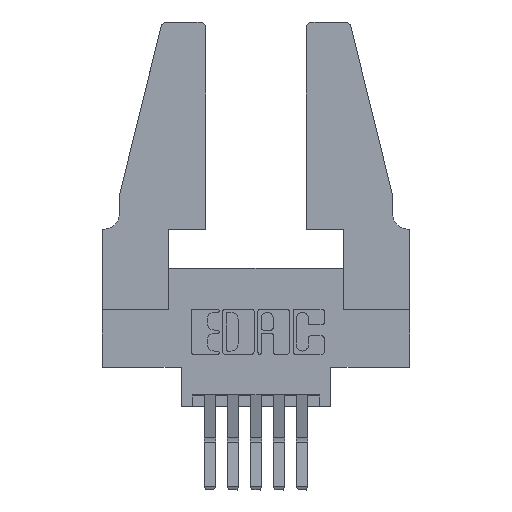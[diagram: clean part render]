
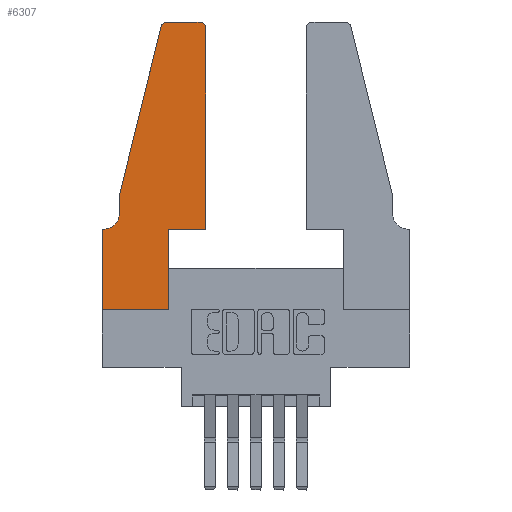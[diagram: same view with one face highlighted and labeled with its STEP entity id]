
A CAD part, top view. The second image highlights one B-rep face of the part: STEP entity #6307.
In plain terms, the highlighted planar face has unit normal (0, 0, 1).
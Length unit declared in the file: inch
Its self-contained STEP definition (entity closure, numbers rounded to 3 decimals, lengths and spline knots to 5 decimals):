
#401 = LINE ( 'NONE', #994, #9424 ) ;
#430 = VERTEX_POINT ( 'NONE', #8927 ) ;
#494 = VERTEX_POINT ( 'NONE', #2024 ) ;
#522 = CARTESIAN_POINT ( 'NONE',  ( 0.0755, 0.5, 0.37 ) ) ;
#534 = EDGE_CURVE ( 'NONE', #494, #732, #2366, .T. ) ;
#602 = CARTESIAN_POINT ( 'NONE',  ( 0.0755, 0.5, 0.37 ) ) ;
#732 = VERTEX_POINT ( 'NONE', #6600 ) ;
#889 = CARTESIAN_POINT ( 'NONE',  ( 0., 0., 0.37 ) ) ;
#952 = EDGE_CURVE ( 'NONE', #11225, #2817, #4703, .T. ) ;
#994 = CARTESIAN_POINT ( 'NONE',  ( 0.2605, 1.25, 0.37 ) ) ;
#1183 = CARTESIAN_POINT ( 'NONE',  ( 0., 0.35, 0.37 ) ) ;
#1318 = EDGE_CURVE ( 'NONE', #732, #4500, #10304, .T. ) ;
#1657 = ORIENTED_EDGE ( 'NONE', *, *, #7045, .T. ) ;
#1787 = DIRECTION ( 'NONE',  ( -1., 0., 0. ) ) ;
#1921 = DIRECTION ( 'NONE',  ( -1., 0., 0. ) ) ;
#1970 = VECTOR ( 'NONE', #2753, 39.37008 ) ;
#2024 = CARTESIAN_POINT ( 'NONE',  ( 0.0055, 0.35, 0.37 ) ) ;
#2245 = ORIENTED_EDGE ( 'NONE', *, *, #534, .T. ) ;
#2366 = LINE ( 'NONE', #7847, #11235 ) ;
#2430 = DIRECTION ( 'NONE',  ( 1., 0., 0. ) ) ;
#2753 = DIRECTION ( 'NONE',  ( 1., 0., 0. ) ) ;
#2759 = VERTEX_POINT ( 'NONE', #7954 ) ;
#2770 = CARTESIAN_POINT ( 'NONE',  ( 0.4505, 1.22, 0.37 ) ) ;
#2807 = AXIS2_PLACEMENT_3D ( 'NONE', #8177, #3059, #9028 ) ;
#2809 = ORIENTED_EDGE ( 'NONE', *, *, #9688, .T. ) ;
#2817 = VERTEX_POINT ( 'NONE', #7139 ) ;
#2929 = LINE ( 'NONE', #602, #4438 ) ;
#2940 = LINE ( 'NONE', #3236, #4973 ) ;
#3044 = DIRECTION ( 'NONE',  ( 0., 0., 1. ) ) ;
#3059 = DIRECTION ( 'NONE',  ( 0., 0., -1. ) ) ;
#3088 = DIRECTION ( 'NONE',  ( 0., 0., 1. ) ) ;
#3107 = LINE ( 'NONE', #4542, #5120 ) ;
#3236 = CARTESIAN_POINT ( 'NONE',  ( 0.2865, 0.35, 0.37 ) ) ;
#3252 = DIRECTION ( 'NONE',  ( 0., 1., 0. ) ) ;
#3321 = DIRECTION ( 'NONE',  ( -0.239, -0.971, 0. ) ) ;
#3409 = EDGE_CURVE ( 'NONE', #2759, #3925, #9166, .T. ) ;
#3623 = FACE_OUTER_BOUND ( 'NONE', #10548, .T. ) ;
#3715 = CARTESIAN_POINT ( 'NONE',  ( 0., 0., 0.37 ) ) ;
#3820 = ORIENTED_EDGE ( 'NONE', *, *, #952, .T. ) ;
#3827 = EDGE_CURVE ( 'NONE', #7275, #11225, #401, .T. ) ;
#3925 = VERTEX_POINT ( 'NONE', #2770 ) ;
#4138 = EDGE_CURVE ( 'NONE', #430, #9712, #2940, .T. ) ;
#4382 = CARTESIAN_POINT ( 'NONE',  ( 0.0755, 0.5, 0.37 ) ) ;
#4438 = VECTOR ( 'NONE', #7618, 39.37008 ) ;
#4500 = VERTEX_POINT ( 'NONE', #9816 ) ;
#4542 = CARTESIAN_POINT ( 'NONE',  ( 0.4505, 0.35, 0.37 ) ) ;
#4644 = VECTOR ( 'NONE', #9183, 39.37008 ) ;
#4703 = CIRCLE ( 'NONE', #6065, 0.03 ) ;
#4973 = VECTOR ( 'NONE', #3252, 39.37008 ) ;
#5120 = VECTOR ( 'NONE', #9648, 39.37008 ) ;
#5141 = CARTESIAN_POINT ( 'NONE',  ( 0.284, 1.22, 0.37 ) ) ;
#5285 = EDGE_CURVE ( 'NONE', #6671, #7124, #2929, .T. ) ;
#5353 = CARTESIAN_POINT ( 'NONE',  ( 0.4505, 0.35, 0.37 ) ) ;
#5599 = CIRCLE ( 'NONE', #10976, 0.03 ) ;
#5601 = PLANE ( 'NONE',  #10428 ) ;
#5956 = CARTESIAN_POINT ( 'NONE',  ( 0.0755, 0.42, 0.37 ) ) ;
#6065 = AXIS2_PLACEMENT_3D ( 'NONE', #5141, #9351, #2430 ) ;
#6307 = ADVANCED_FACE ( 'NONE', ( #3623 ), #5601, .T. ) ;
#6325 = EDGE_CURVE ( 'NONE', #3925, #7275, #5599, .T. ) ;
#6600 = CARTESIAN_POINT ( 'NONE',  ( 0., 0.35, 0.37 ) ) ;
#6671 = VERTEX_POINT ( 'NONE', #4382 ) ;
#6820 = ORIENTED_EDGE ( 'NONE', *, *, #1318, .T. ) ;
#6933 = CARTESIAN_POINT ( 'NONE',  ( 0.4205, 1.25, 0.37 ) ) ;
#7045 = EDGE_CURVE ( 'NONE', #2817, #6671, #11178, .T. ) ;
#7097 = ORIENTED_EDGE ( 'NONE', *, *, #4138, .T. ) ;
#7124 = VERTEX_POINT ( 'NONE', #5956 ) ;
#7139 = CARTESIAN_POINT ( 'NONE',  ( 0.25487, 1.22718, 0.37 ) ) ;
#7272 = CARTESIAN_POINT ( 'NONE',  ( 0.284, 1.25, 0.37 ) ) ;
#7275 = VERTEX_POINT ( 'NONE', #6933 ) ;
#7373 = ORIENTED_EDGE ( 'NONE', *, *, #3409, .T. ) ;
#7618 = DIRECTION ( 'NONE',  ( 0., -1., 0. ) ) ;
#7630 = ORIENTED_EDGE ( 'NONE', *, *, #6325, .T. ) ;
#7812 = CIRCLE ( 'NONE', #2807, 0.07 ) ;
#7847 = CARTESIAN_POINT ( 'NONE',  ( 0.0755, 0.35, 0.37 ) ) ;
#7954 = CARTESIAN_POINT ( 'NONE',  ( 0.4505, 0.35, 0.37 ) ) ;
#8007 = VECTOR ( 'NONE', #9663, 39.37008 ) ;
#8035 = ORIENTED_EDGE ( 'NONE', *, *, #3827, .T. ) ;
#8038 = EDGE_CURVE ( 'NONE', #7124, #494, #7812, .T. ) ;
#8177 = CARTESIAN_POINT ( 'NONE',  ( 0.0055, 0.42, 0.37 ) ) ;
#8203 = CARTESIAN_POINT ( 'NONE',  ( 0.4205, 1.22, 0.37 ) ) ;
#8839 = ORIENTED_EDGE ( 'NONE', *, *, #8038, .T. ) ;
#8903 = VECTOR ( 'NONE', #3321, 39.37008 ) ;
#8927 = CARTESIAN_POINT ( 'NONE',  ( 0.2865, 0., 0.37 ) ) ;
#9020 = DIRECTION ( 'NONE',  ( 1., 0., 0. ) ) ;
#9028 = DIRECTION ( 'NONE',  ( -1., 0., 0. ) ) ;
#9056 = DIRECTION ( 'NONE',  ( 1., 0., 0. ) ) ;
#9109 = ORIENTED_EDGE ( 'NONE', *, *, #10422, .T. ) ;
#9166 = LINE ( 'NONE', #5353, #4644 ) ;
#9183 = DIRECTION ( 'NONE',  ( 0., 1., 0. ) ) ;
#9351 = DIRECTION ( 'NONE',  ( 0., 0., 1. ) ) ;
#9424 = VECTOR ( 'NONE', #1921, 39.37008 ) ;
#9648 = DIRECTION ( 'NONE',  ( 1., 0., 0. ) ) ;
#9663 = DIRECTION ( 'NONE',  ( 0., -1., 0. ) ) ;
#9687 = CARTESIAN_POINT ( 'NONE',  ( 0.2865, 0.35, 0.37 ) ) ;
#9688 = EDGE_CURVE ( 'NONE', #9712, #2759, #3107, .T. ) ;
#9712 = VERTEX_POINT ( 'NONE', #9687 ) ;
#9816 = CARTESIAN_POINT ( 'NONE',  ( 0., 0., 0.37 ) ) ;
#10304 = LINE ( 'NONE', #3715, #8007 ) ;
#10422 = EDGE_CURVE ( 'NONE', #4500, #430, #11131, .T. ) ;
#10428 = AXIS2_PLACEMENT_3D ( 'NONE', #1183, #3044, #9020 ) ;
#10548 = EDGE_LOOP ( 'NONE', ( #8035, #3820, #1657, #10859, #8839, #2245, #6820, #9109, #7097, #2809, #7373, #7630 ) ) ;
#10859 = ORIENTED_EDGE ( 'NONE', *, *, #5285, .T. ) ;
#10976 = AXIS2_PLACEMENT_3D ( 'NONE', #8203, #3088, #9056 ) ;
#11131 = LINE ( 'NONE', #889, #1970 ) ;
#11178 = LINE ( 'NONE', #522, #8903 ) ;
#11225 = VERTEX_POINT ( 'NONE', #7272 ) ;
#11235 = VECTOR ( 'NONE', #1787, 39.37008 ) ;
